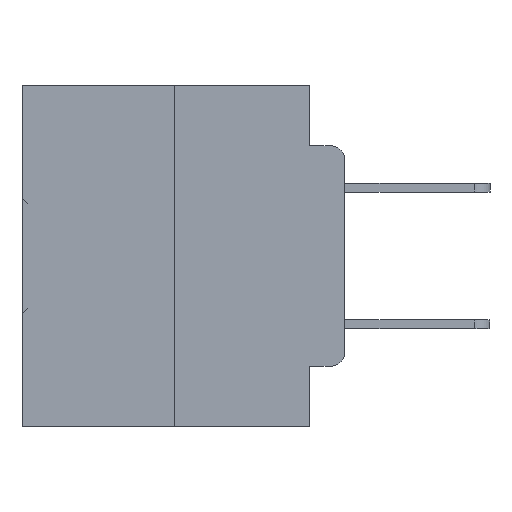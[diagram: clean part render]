
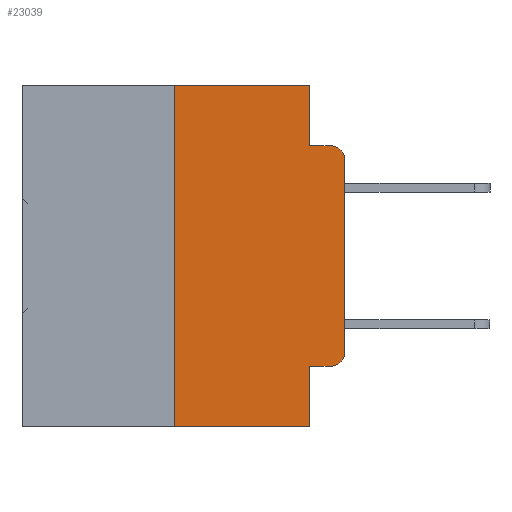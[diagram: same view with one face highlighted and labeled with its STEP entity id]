
A CAD part, left-side view. The second image highlights one B-rep face of the part: STEP entity #23039.
In plain terms, the highlighted planar face has unit normal (-1, 0, 0).
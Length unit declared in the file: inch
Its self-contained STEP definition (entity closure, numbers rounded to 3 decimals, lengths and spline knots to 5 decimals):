
#227 = CARTESIAN_POINT ( 'NONE',  ( 0., 0.051, -0.4115 ) ) ;
#258 = VECTOR ( 'NONE', #16843, 39.37008 ) ;
#463 = DIRECTION ( 'NONE',  ( 0., 0., -1. ) ) ;
#509 = ORIENTED_EDGE ( 'NONE', *, *, #29477, .F. ) ;
#1154 = CARTESIAN_POINT ( 'NONE',  ( 0., 0.25, 0. ) ) ;
#1157 = VERTEX_POINT ( 'NONE', #22322 ) ;
#1324 = DIRECTION ( 'NONE',  ( -1., 0., 0. ) ) ;
#1740 = VERTEX_POINT ( 'NONE', #14370 ) ;
#2604 = ORIENTED_EDGE ( 'NONE', *, *, #28620, .T. ) ;
#2923 = DIRECTION ( 'NONE',  ( 0., -1., 0. ) ) ;
#3813 = DIRECTION ( 'NONE',  ( 0., 0., -1. ) ) ;
#4300 = ORIENTED_EDGE ( 'NONE', *, *, #30786, .F. ) ;
#4391 = CARTESIAN_POINT ( 'NONE',  ( 0., 0.25, -0.5 ) ) ;
#4551 = CARTESIAN_POINT ( 'NONE',  ( 0., 0.051, -0.0885 ) ) ;
#4586 = EDGE_CURVE ( 'NONE', #15069, #29682, #20662, .T. ) ;
#5589 = ORIENTED_EDGE ( 'NONE', *, *, #18412, .T. ) ;
#5653 = CARTESIAN_POINT ( 'NONE',  ( 0., 0.051, 0. ) ) ;
#5933 = VECTOR ( 'NONE', #2923, 39.37008 ) ;
#5990 = ORIENTED_EDGE ( 'NONE', *, *, #28054, .F. ) ;
#6531 = CIRCLE ( 'NONE', #25703, 0.02 ) ;
#6681 = DIRECTION ( 'NONE',  ( 0., 0., 1. ) ) ;
#7227 = ORIENTED_EDGE ( 'NONE', *, *, #4586, .T. ) ;
#7424 = LINE ( 'NONE', #11446, #258 ) ;
#8589 = VERTEX_POINT ( 'NONE', #32133 ) ;
#9202 = CIRCLE ( 'NONE', #27376, 0.02 ) ;
#9264 = FACE_OUTER_BOUND ( 'NONE', #26790, .T. ) ;
#9478 = VERTEX_POINT ( 'NONE', #4391 ) ;
#9728 = LINE ( 'NONE', #1154, #30261 ) ;
#9913 = DIRECTION ( 'NONE',  ( 1., 0., 0. ) ) ;
#10607 = EDGE_CURVE ( 'NONE', #32921, #32346, #27319, .T. ) ;
#10761 = VECTOR ( 'NONE', #3813, 39.37008 ) ;
#11117 = CARTESIAN_POINT ( 'NONE',  ( 0., 0., -0.1085 ) ) ;
#11362 = CARTESIAN_POINT ( 'NONE',  ( 0., 0.051, -0.4115 ) ) ;
#11446 = CARTESIAN_POINT ( 'NONE',  ( 0., 0.051, 0. ) ) ;
#14370 = CARTESIAN_POINT ( 'NONE',  ( 0., 0.25, 0. ) ) ;
#15069 = VERTEX_POINT ( 'NONE', #25099 ) ;
#16169 = AXIS2_PLACEMENT_3D ( 'NONE', #25991, #9913, #28664 ) ;
#16589 = DIRECTION ( 'NONE',  ( -1., 0., 0. ) ) ;
#16843 = DIRECTION ( 'NONE',  ( 0., 0., -1. ) ) ;
#17434 = CARTESIAN_POINT ( 'NONE',  ( 0., 0.02, -0.1085 ) ) ;
#17821 = DIRECTION ( 'NONE',  ( 0., 0., 1. ) ) ;
#17937 = LINE ( 'NONE', #30503, #10761 ) ;
#17940 = EDGE_CURVE ( 'NONE', #9478, #1740, #9728, .T. ) ;
#17979 = LINE ( 'NONE', #30414, #31288 ) ;
#18412 = EDGE_CURVE ( 'NONE', #9478, #32702, #17979, .T. ) ;
#18980 = EDGE_CURVE ( 'NONE', #32921, #32702, #7424, .T. ) ;
#20131 = DIRECTION ( 'NONE',  ( 0., 0., -1. ) ) ;
#20662 = LINE ( 'NONE', #34585, #33886 ) ;
#20784 = VECTOR ( 'NONE', #21015, 39.37008 ) ;
#21015 = DIRECTION ( 'NONE',  ( 0., -1., 0. ) ) ;
#22322 = CARTESIAN_POINT ( 'NONE',  ( 0., 0.051, -0.0885 ) ) ;
#23039 = ADVANCED_FACE ( 'NONE', ( #9264 ), #25890, .F. ) ;
#23290 = ORIENTED_EDGE ( 'NONE', *, *, #10607, .T. ) ;
#23393 = DIRECTION ( 'NONE',  ( 0., -1., 0. ) ) ;
#23919 = EDGE_CURVE ( 'NONE', #32346, #15069, #9202, .T. ) ;
#24518 = ORIENTED_EDGE ( 'NONE', *, *, #17940, .F. ) ;
#25099 = CARTESIAN_POINT ( 'NONE',  ( 0., 0., -0.3915 ) ) ;
#25703 = AXIS2_PLACEMENT_3D ( 'NONE', #17434, #1324, #20131 ) ;
#25890 = PLANE ( 'NONE',  #16169 ) ;
#25991 = CARTESIAN_POINT ( 'NONE',  ( 0., 0.473, 0. ) ) ;
#26790 = EDGE_LOOP ( 'NONE', ( #7227, #2604, #4300, #5990, #509, #24518, #5589, #27828, #23290, #31121 ) ) ;
#27319 = LINE ( 'NONE', #227, #5933 ) ;
#27376 = AXIS2_PLACEMENT_3D ( 'NONE', #32521, #16589, #463 ) ;
#27769 = LINE ( 'NONE', #4551, #28582 ) ;
#27770 = DIRECTION ( 'NONE',  ( 0., -1., 0. ) ) ;
#27828 = ORIENTED_EDGE ( 'NONE', *, *, #18980, .F. ) ;
#27870 = LINE ( 'NONE', #31575, #20784 ) ;
#28054 = EDGE_CURVE ( 'NONE', #29007, #1157, #17937, .T. ) ;
#28582 = VECTOR ( 'NONE', #23393, 39.37008 ) ;
#28620 = EDGE_CURVE ( 'NONE', #29682, #8589, #6531, .T. ) ;
#28664 = DIRECTION ( 'NONE',  ( 0., 0., -1. ) ) ;
#29007 = VERTEX_POINT ( 'NONE', #5653 ) ;
#29477 = EDGE_CURVE ( 'NONE', #1740, #29007, #27870, .T. ) ;
#29682 = VERTEX_POINT ( 'NONE', #11117 ) ;
#30261 = VECTOR ( 'NONE', #6681, 39.37008 ) ;
#30334 = CARTESIAN_POINT ( 'NONE',  ( 0., 0.02, -0.4115 ) ) ;
#30414 = CARTESIAN_POINT ( 'NONE',  ( 0., 0.473, -0.5 ) ) ;
#30503 = CARTESIAN_POINT ( 'NONE',  ( 0., 0.051, 0. ) ) ;
#30786 = EDGE_CURVE ( 'NONE', #1157, #8589, #27769, .T. ) ;
#31121 = ORIENTED_EDGE ( 'NONE', *, *, #23919, .T. ) ;
#31288 = VECTOR ( 'NONE', #27770, 39.37008 ) ;
#31575 = CARTESIAN_POINT ( 'NONE',  ( 0., 0.473, 0. ) ) ;
#31797 = CARTESIAN_POINT ( 'NONE',  ( 0., 0.051, -0.5 ) ) ;
#32133 = CARTESIAN_POINT ( 'NONE',  ( 0., 0.02, -0.0885 ) ) ;
#32346 = VERTEX_POINT ( 'NONE', #30334 ) ;
#32521 = CARTESIAN_POINT ( 'NONE',  ( 0., 0.02, -0.3915 ) ) ;
#32702 = VERTEX_POINT ( 'NONE', #31797 ) ;
#32921 = VERTEX_POINT ( 'NONE', #11362 ) ;
#33886 = VECTOR ( 'NONE', #17821, 39.37008 ) ;
#34585 = CARTESIAN_POINT ( 'NONE',  ( 0., 0., 0. ) ) ;
